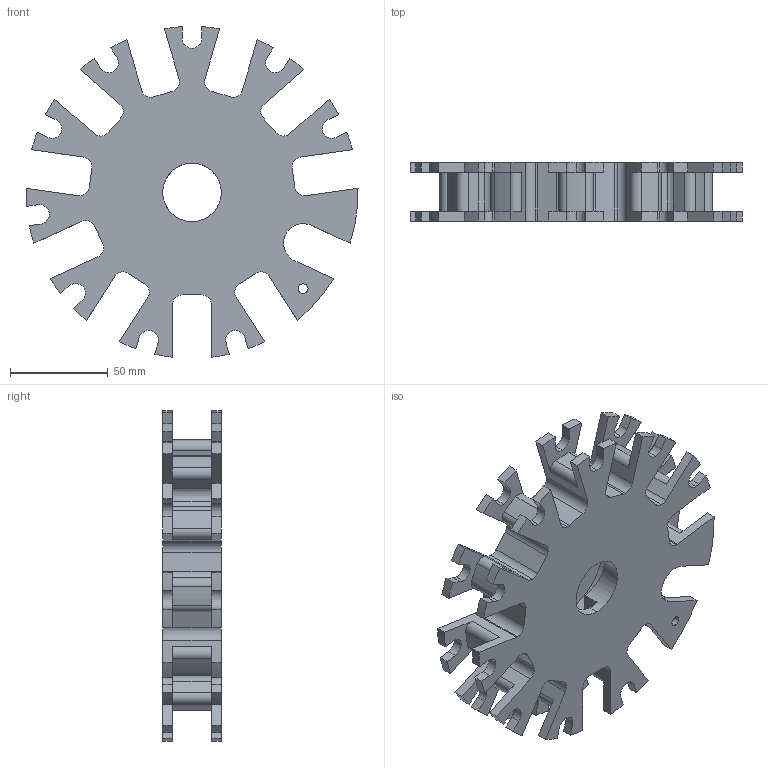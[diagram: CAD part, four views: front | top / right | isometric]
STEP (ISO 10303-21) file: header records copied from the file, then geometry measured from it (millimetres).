
FILE_DESCRIPTION (( 'STEP AP214' ), '1' );
FILE_NAME ('spindle.STEP', '2013-12-22T02:50:57', ( '' ), ( '' ), 'SwSTEP 2.0', 'SolidWorks 2013', '' );
FILE_SCHEMA (( 'AUTOMOTIVE_DESIGN' ));
Length unit declared in the file: millimetre
Products named in the file (1): spindle
Bounding box: 169.97 x 30 x 169.26 mm (x, y, z)
Volume: 324716.5 mm3; surface area: 70680.5 mm2
Topology: 1 solids, 1 shells, 252 faces, 743 edges, 493 vertices
Faces by surface type: cylinder 146, plane 102, bspline 4
Entity records: 8774 total; most frequent: CARTESIAN_POINT 1745, DIRECTION 1530, ORIENTED_EDGE 1486, EDGE_CURVE 743, AXIS2_PLACEMENT_3D 545, VERTEX_POINT 493, LINE 440, VECTOR 440
